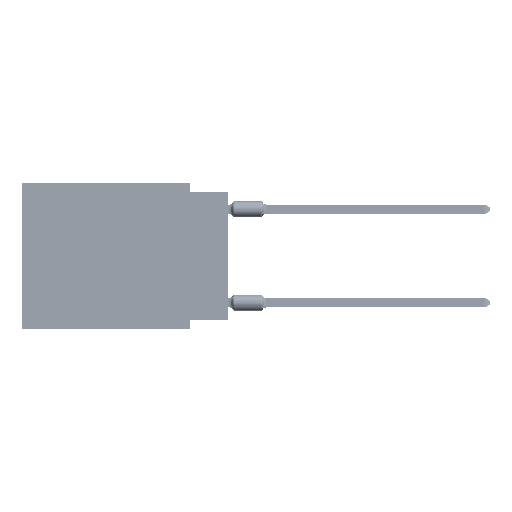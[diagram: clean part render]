
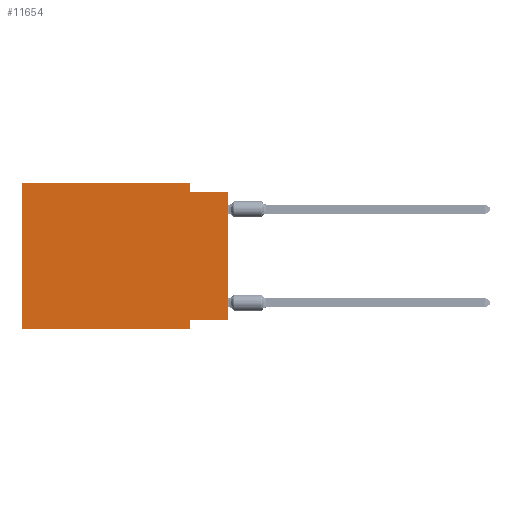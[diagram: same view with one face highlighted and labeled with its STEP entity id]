
A CAD part, left-side view. The second image highlights one B-rep face of the part: STEP entity #11654.
In plain terms, the highlighted planar face has unit normal (-1, 0, 0).
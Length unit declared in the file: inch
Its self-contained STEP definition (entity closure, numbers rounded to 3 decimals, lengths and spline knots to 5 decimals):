
#822 = DIRECTION ( 'NONE',  ( 0., 0., -1. ) ) ;
#3235 = EDGE_CURVE ( 'NONE', #59570, #60019, #64990, .T. ) ;
#3394 = VECTOR ( 'NONE', #51414, 39.37008 ) ;
#4018 = EDGE_CURVE ( 'NONE', #17899, #66365, #52111, .T. ) ;
#4062 = VERTEX_POINT ( 'NONE', #54168 ) ;
#5665 = CARTESIAN_POINT ( 'NONE',  ( 0., 0.1, -0.025 ) ) ;
#6536 = ORIENTED_EDGE ( 'NONE', *, *, #22551, .F. ) ;
#7265 = CARTESIAN_POINT ( 'NONE',  ( 0., 0.55, 0. ) ) ;
#7697 = CARTESIAN_POINT ( 'NONE',  ( 0., 0.1, 0. ) ) ;
#9211 = PLANE ( 'NONE',  #33727 ) ;
#9722 = CARTESIAN_POINT ( 'NONE',  ( 0., 0.1, -0.39 ) ) ;
#10920 = ORIENTED_EDGE ( 'NONE', *, *, #40105, .F. ) ;
#11193 = VECTOR ( 'NONE', #44990, 39.37008 ) ;
#11654 = ADVANCED_FACE ( 'NONE', ( #53175 ), #9211, .F. ) ;
#12875 = CARTESIAN_POINT ( 'NONE',  ( 0., 0.55, -0.39 ) ) ;
#13433 = VECTOR ( 'NONE', #14228, 39.37008 ) ;
#13847 = ORIENTED_EDGE ( 'NONE', *, *, #23270, .F. ) ;
#13938 = DIRECTION ( 'NONE',  ( 1., 0., 0. ) ) ;
#14228 = DIRECTION ( 'NONE',  ( 0., 0., -1. ) ) ;
#15018 = CARTESIAN_POINT ( 'NONE',  ( 0., 0.55, 0. ) ) ;
#15387 = LINE ( 'NONE', #65535, #65915 ) ;
#15769 = VERTEX_POINT ( 'NONE', #50443 ) ;
#16790 = ORIENTED_EDGE ( 'NONE', *, *, #3235, .F. ) ;
#17445 = ORIENTED_EDGE ( 'NONE', *, *, #56052, .F. ) ;
#17899 = VERTEX_POINT ( 'NONE', #12875 ) ;
#19531 = CARTESIAN_POINT ( 'NONE',  ( 0., 0.55, -0.39 ) ) ;
#22441 = CARTESIAN_POINT ( 'NONE',  ( 0., 0.1, 0. ) ) ;
#22551 = EDGE_CURVE ( 'NONE', #15769, #66961, #24745, .T. ) ;
#23270 = EDGE_CURVE ( 'NONE', #4062, #15769, #51498, .T. ) ;
#24160 = LINE ( 'NONE', #35072, #46256 ) ;
#24745 = LINE ( 'NONE', #70178, #13433 ) ;
#27345 = DIRECTION ( 'NONE',  ( 0., 0., 1. ) ) ;
#33727 = AXIS2_PLACEMENT_3D ( 'NONE', #15018, #13938, #57537 ) ;
#34043 = VECTOR ( 'NONE', #822, 39.37008 ) ;
#34161 = ORIENTED_EDGE ( 'NONE', *, *, #50511, .T. ) ;
#34252 = CARTESIAN_POINT ( 'NONE',  ( 0., 0., -0.025 ) ) ;
#35072 = CARTESIAN_POINT ( 'NONE',  ( 0., 0.55, 0. ) ) ;
#40105 = EDGE_CURVE ( 'NONE', #66365, #41274, #24160, .T. ) ;
#40563 = CARTESIAN_POINT ( 'NONE',  ( 0., 0., -0.365 ) ) ;
#41274 = VERTEX_POINT ( 'NONE', #22441 ) ;
#41317 = VECTOR ( 'NONE', #70444, 39.37008 ) ;
#42062 = LINE ( 'NONE', #19531, #55752 ) ;
#44990 = DIRECTION ( 'NONE',  ( 0., 1., 0. ) ) ;
#45942 = CARTESIAN_POINT ( 'NONE',  ( 0., 0.55, 0. ) ) ;
#46256 = VECTOR ( 'NONE', #46724, 39.37008 ) ;
#46724 = DIRECTION ( 'NONE',  ( 0., -1., 0. ) ) ;
#47037 = EDGE_CURVE ( 'NONE', #4062, #60019, #15387, .T. ) ;
#50443 = CARTESIAN_POINT ( 'NONE',  ( 0., 0.1, -0.365 ) ) ;
#50511 = EDGE_CURVE ( 'NONE', #17899, #66961, #42062, .T. ) ;
#50979 = LINE ( 'NONE', #7697, #34043 ) ;
#51414 = DIRECTION ( 'NONE',  ( 0., 0., 1. ) ) ;
#51498 = LINE ( 'NONE', #40563, #11193 ) ;
#52111 = LINE ( 'NONE', #45942, #3394 ) ;
#53175 = FACE_OUTER_BOUND ( 'NONE', #57364, .T. ) ;
#53357 = CARTESIAN_POINT ( 'NONE',  ( 0., 0., -0.025 ) ) ;
#54168 = CARTESIAN_POINT ( 'NONE',  ( 0., 0., -0.365 ) ) ;
#55752 = VECTOR ( 'NONE', #64237, 39.37008 ) ;
#56052 = EDGE_CURVE ( 'NONE', #41274, #59570, #50979, .T. ) ;
#57364 = EDGE_LOOP ( 'NONE', ( #60402, #16790, #17445, #10920, #69520, #34161, #6536, #13847 ) ) ;
#57537 = DIRECTION ( 'NONE',  ( 0., 0., -1. ) ) ;
#59570 = VERTEX_POINT ( 'NONE', #5665 ) ;
#60019 = VERTEX_POINT ( 'NONE', #34252 ) ;
#60402 = ORIENTED_EDGE ( 'NONE', *, *, #47037, .T. ) ;
#64237 = DIRECTION ( 'NONE',  ( 0., -1., 0. ) ) ;
#64990 = LINE ( 'NONE', #53357, #41317 ) ;
#65535 = CARTESIAN_POINT ( 'NONE',  ( 0., 0., 0. ) ) ;
#65915 = VECTOR ( 'NONE', #27345, 39.37008 ) ;
#66365 = VERTEX_POINT ( 'NONE', #7265 ) ;
#66961 = VERTEX_POINT ( 'NONE', #9722 ) ;
#69520 = ORIENTED_EDGE ( 'NONE', *, *, #4018, .F. ) ;
#70178 = CARTESIAN_POINT ( 'NONE',  ( 0., 0.1, -0.39 ) ) ;
#70444 = DIRECTION ( 'NONE',  ( 0., -1., 0. ) ) ;
